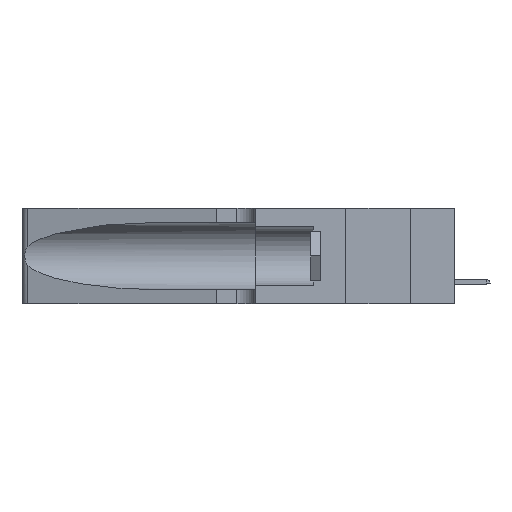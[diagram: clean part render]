
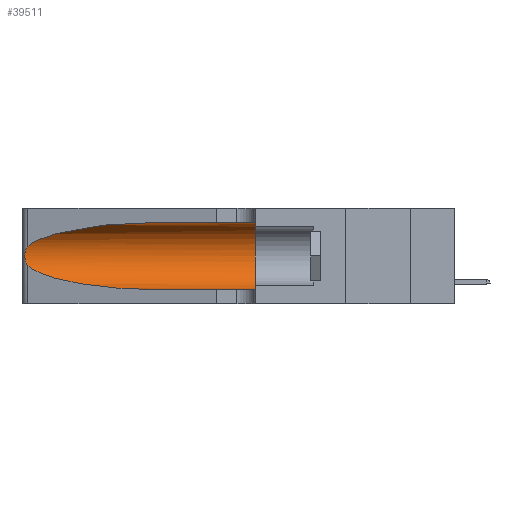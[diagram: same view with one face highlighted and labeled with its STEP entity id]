
A CAD part, left-side view. The second image highlights one B-rep face of the part: STEP entity #39511.
In plain terms, the highlighted cylindrical face has radius 3.308 mm (diameter 6.617 mm), a partial arc.
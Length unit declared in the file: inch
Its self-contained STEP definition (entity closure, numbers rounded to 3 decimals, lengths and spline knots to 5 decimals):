
#85 = CARTESIAN_POINT ( 'NONE',  ( 0.26018, 1.23835, 0.19895 ) ) ;
#772 = CARTESIAN_POINT ( 'NONE',  ( 0.25854, 1.2359, 0.20912 ) ) ;
#1507 = EDGE_CURVE ( 'NONE', #10719, #41362, #6779, .T. ) ;
#1928 = CARTESIAN_POINT ( 'NONE',  ( 0.2373, 1.15595, 0.28018 ) ) ;
#3187 = DIRECTION ( 'NONE',  ( 0., 1., 0. ) ) ;
#4300 = CARTESIAN_POINT ( 'NONE',  ( 0.18966, 0.96281, 0.31525 ) ) ;
#4438 = CARTESIAN_POINT ( 'NONE',  ( 0.1305, 0.72297, 0.05475 ) ) ;
#4506 = CARTESIAN_POINT ( 'NONE',  ( 0.26017, 1.23833, 0.17102 ) ) ;
#5209 = CARTESIAN_POINT ( 'NONE',  ( 0.1305, 0.72297, 0.31525 ) ) ;
#6564 = CIRCLE ( 'NONE', #16302, 0.13025 ) ;
#6779 = LINE ( 'NONE', #25277, #30338 ) ;
#8440 = CARTESIAN_POINT ( 'NONE',  ( 0.1305, 0.72297, 0.31525 ) ) ;
#9250 = AXIS2_PLACEMENT_3D ( 'NONE', #31229, #14117, #28412 ) ;
#9523 = ORIENTED_EDGE ( 'NONE', *, *, #45234, .F. ) ;
#10719 = VERTEX_POINT ( 'NONE', #8440 ) ;
#13630 = ORIENTED_EDGE ( 'NONE', *, *, #19721, .T. ) ;
#13944 = DIRECTION ( 'NONE',  ( 0., 0., 1. ) ) ;
#14117 = DIRECTION ( 'NONE',  ( 0., -1., 0. ) ) ;
#14348 = CARTESIAN_POINT ( 'NONE',  ( 0.25555, 1.22993, 0.14849 ) ) ;
#14824 = CARTESIAN_POINT ( 'NONE',  ( 0.25555, 1.22994, 0.2215 ) ) ;
#16255 = EDGE_LOOP ( 'NONE', ( #13630, #36807, #41050, #22449, #9523, #38894 ) ) ;
#16302 = AXIS2_PLACEMENT_3D ( 'NONE', #35312, #3187, #13944 ) ;
#16671 = CARTESIAN_POINT ( 'NONE',  ( 0.25487, 1.22718, 0.14631 ) ) ;
#16898 = CARTESIAN_POINT ( 'NONE',  ( 0.1305, 0.72297, 0.05475 ) ) ;
#17570 = LINE ( 'NONE', #45744, #36515 ) ;
#18542 = CARTESIAN_POINT ( 'NONE',  ( 0.26075, 1.23896, 0.19203 ) ) ;
#18772 = CARTESIAN_POINT ( 'NONE',  ( 0.25856, 1.23593, 0.16098 ) ) ;
#19721 = EDGE_CURVE ( 'NONE', #10719, #20171, #45837, .T. ) ;
#19821 = EDGE_CURVE ( 'NONE', #22562, #40819, #34452, .T. ) ;
#20171 = VERTEX_POINT ( 'NONE', #41951 ) ;
#22449 = ORIENTED_EDGE ( 'NONE', *, *, #44742, .T. ) ;
#22562 = VERTEX_POINT ( 'NONE', #39036 ) ;
#23681 = CARTESIAN_POINT ( 'NONE',  ( 0.18966, 0.96281, 0.05475 ) ) ;
#24653 = CARTESIAN_POINT ( 'NONE',  ( 0.1305, 0.35, 0.31525 ) ) ;
#25277 = CARTESIAN_POINT ( 'NONE',  ( 0.1305, 1.61858, 0.31525 ) ) ;
#25580 = CARTESIAN_POINT ( 'NONE',  ( 0.25487, 1.22718, 0.22369 ) ) ;
#27203 = CARTESIAN_POINT ( 'NONE',  ( 0.25487, 1.22718, 0.22369 ) ) ;
#28412 = DIRECTION ( 'NONE',  ( 0., 0., -1. ) ) ;
#28658 = CARTESIAN_POINT ( 'NONE',  ( 0.25487, 1.22718, 0.14631 ) ) ;
#29560 = CARTESIAN_POINT ( 'NONE',  ( 0.25639, 1.23186, 0.15144 ) ) ;
#30338 = VECTOR ( 'NONE', #46202, 39.37008 ) ;
#31229 = CARTESIAN_POINT ( 'NONE',  ( 0.1305, 1.61858, 0.185 ) ) ;
#32855 = CARTESIAN_POINT ( 'NONE',  ( 0.1305, 0.35, 0.05475 ) ) ;
#32865 = CARTESIAN_POINT ( 'NONE',  ( 0.26075, 1.23896, 0.178 ) ) ;
#33098 = CARTESIAN_POINT ( 'NONE',  ( 0.25789, 1.23486, 0.15765 ) ) ;
#34452 =( BOUNDED_CURVE ( )  B_SPLINE_CURVE ( 3, ( #16671, #41540, #23681, #16898 ),
 .UNSPECIFIED., .F., .T. ) 
 B_SPLINE_CURVE_WITH_KNOTS ( ( 4, 4 ),
 ( 3.44316, 4.71239 ),
 .UNSPECIFIED. ) 
 CURVE ( )  GEOMETRIC_REPRESENTATION_ITEM ( )  RATIONAL_B_SPLINE_CURVE ( ( 1., 0.87, 0.87, 1. ) ) 
 REPRESENTATION_ITEM ( '' )  );
#35312 = CARTESIAN_POINT ( 'NONE',  ( 0.1305, 0.35, 0.185 ) ) ;
#36515 = VECTOR ( 'NONE', #38712, 39.37008 ) ;
#36807 = ORIENTED_EDGE ( 'NONE', *, *, #39590, .T. ) ;
#38306 = CYLINDRICAL_SURFACE ( 'NONE', #9250, 0.13025 ) ;
#38712 = DIRECTION ( 'NONE',  ( 0., -1., 0. ) ) ;
#38894 = ORIENTED_EDGE ( 'NONE', *, *, #1507, .F. ) ;
#39036 = CARTESIAN_POINT ( 'NONE',  ( 0.25487, 1.22718, 0.14631 ) ) ;
#39471 = CARTESIAN_POINT ( 'NONE',  ( 0.25639, 1.23184, 0.21858 ) ) ;
#39511 = ADVANCED_FACE ( 'NONE', ( #46273 ), #38306, .F. ) ;
#39590 = EDGE_CURVE ( 'NONE', #20171, #22562, #45284, .T. ) ;
#39928 = CARTESIAN_POINT ( 'NONE',  ( 0.25787, 1.23484, 0.2124 ) ) ;
#40278 = VERTEX_POINT ( 'NONE', #32855 ) ;
#40819 = VERTEX_POINT ( 'NONE', #4438 ) ;
#41050 = ORIENTED_EDGE ( 'NONE', *, *, #19821, .T. ) ;
#41362 = VERTEX_POINT ( 'NONE', #24653 ) ;
#41540 = CARTESIAN_POINT ( 'NONE',  ( 0.2373, 1.15595, 0.08982 ) ) ;
#41951 = CARTESIAN_POINT ( 'NONE',  ( 0.25487, 1.22718, 0.22369 ) ) ;
#44742 = EDGE_CURVE ( 'NONE', #40819, #40278, #17570, .T. ) ;
#45234 = EDGE_CURVE ( 'NONE', #41362, #40278, #6564, .T. ) ;
#45284 = B_SPLINE_CURVE_WITH_KNOTS ( 'NONE', 3,
 ( #25580, #14824, #39471, #39928, #772, #85, #18542, #32865, #4506, #18772, #33098, #29560, #14348, #28658 ),
 .UNSPECIFIED., .F., .F.,
 ( 4, 2, 2, 2, 2, 2, 4 ),
 ( 0., 0.00027, 0.00053, 0.00107, 0.0016, 0.00187, 0.00214 ),
 .UNSPECIFIED. ) ;
#45744 = CARTESIAN_POINT ( 'NONE',  ( 0.1305, 1.61858, 0.05475 ) ) ;
#45837 =( BOUNDED_CURVE ( )  B_SPLINE_CURVE ( 3, ( #5209, #4300, #1928, #27203 ),
 .UNSPECIFIED., .F., .T. ) 
 B_SPLINE_CURVE_WITH_KNOTS ( ( 4, 4 ),
 ( 1.5708, 2.84003 ),
 .UNSPECIFIED. ) 
 CURVE ( )  GEOMETRIC_REPRESENTATION_ITEM ( )  RATIONAL_B_SPLINE_CURVE ( ( 1., 0.87, 0.87, 1. ) ) 
 REPRESENTATION_ITEM ( '' )  );
#46202 = DIRECTION ( 'NONE',  ( 0., -1., 0. ) ) ;
#46273 = FACE_OUTER_BOUND ( 'NONE', #16255, .T. ) ;
